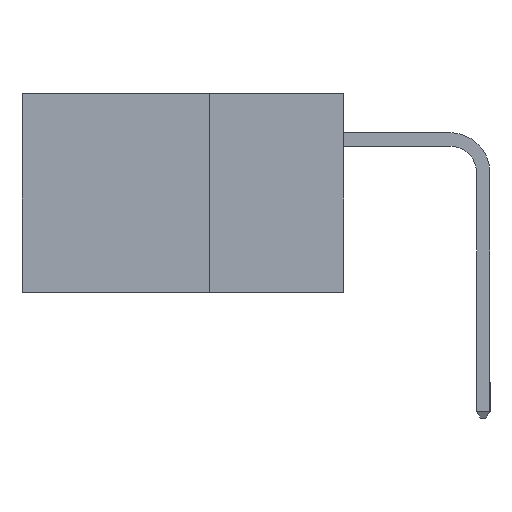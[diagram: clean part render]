
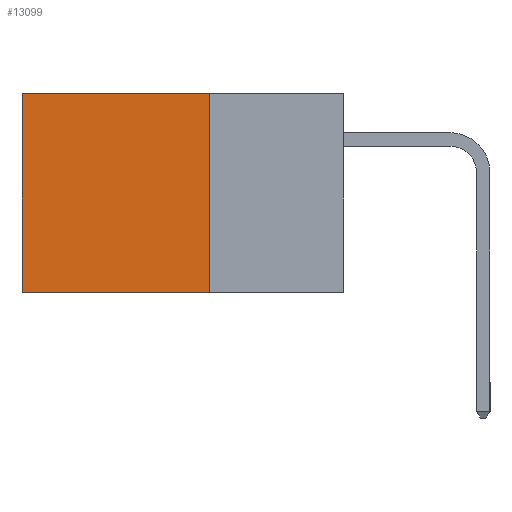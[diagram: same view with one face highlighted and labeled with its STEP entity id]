
A CAD part, left-side view. The second image highlights one B-rep face of the part: STEP entity #13099.
In plain terms, the highlighted planar face has unit normal (-1, 0, 0).
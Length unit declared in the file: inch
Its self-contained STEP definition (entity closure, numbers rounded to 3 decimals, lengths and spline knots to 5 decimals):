
#156 = DIRECTION ( 'NONE',  ( 0., 1., 0. ) ) ;
#207 = ORIENTED_EDGE ( 'NONE', *, *, #7930, .T. ) ;
#436 = ORIENTED_EDGE ( 'NONE', *, *, #2100, .F. ) ;
#729 = ORIENTED_EDGE ( 'NONE', *, *, #3779, .F. ) ;
#1089 = DIRECTION ( 'NONE',  ( 0., 0., -1. ) ) ;
#1371 = AXIS2_PLACEMENT_3D ( 'NONE', #12196, #5214, #13262 ) ;
#2100 = EDGE_CURVE ( 'NONE', #11274, #3250, #14864, .T. ) ;
#2381 = ORIENTED_EDGE ( 'NONE', *, *, #7625, .T. ) ;
#2775 = EDGE_LOOP ( 'NONE', ( #207, #436, #729, #2381 ) ) ;
#3250 = VERTEX_POINT ( 'NONE', #8927 ) ;
#3779 = EDGE_CURVE ( 'NONE', #6844, #11274, #8125, .T. ) ;
#3954 = PLANE ( 'NONE',  #1371 ) ;
#4610 = CARTESIAN_POINT ( 'NONE',  ( 0.298, 0.25, 0. ) ) ;
#5214 = DIRECTION ( 'NONE',  ( 1., 0., 0. ) ) ;
#5579 = CARTESIAN_POINT ( 'NONE',  ( 0.298, 0.6, 0. ) ) ;
#5842 = VECTOR ( 'NONE', #156, 39.37008 ) ;
#6231 = CARTESIAN_POINT ( 'NONE',  ( 0.298, 0.6, 0. ) ) ;
#6844 = VERTEX_POINT ( 'NONE', #4610 ) ;
#7481 = DIRECTION ( 'NONE',  ( 0., 1., 0. ) ) ;
#7625 = EDGE_CURVE ( 'NONE', #6844, #10869, #12028, .T. ) ;
#7738 = VECTOR ( 'NONE', #9317, 39.37008 ) ;
#7930 = EDGE_CURVE ( 'NONE', #10869, #3250, #11678, .T. ) ;
#8125 = LINE ( 'NONE', #10690, #7738 ) ;
#8489 = CARTESIAN_POINT ( 'NONE',  ( 0.298, 0.25, -0.37 ) ) ;
#8927 = CARTESIAN_POINT ( 'NONE',  ( 0.298, 0.6, -0.37 ) ) ;
#9141 = CARTESIAN_POINT ( 'NONE',  ( 0.298, 0.25, 0. ) ) ;
#9213 = VECTOR ( 'NONE', #7481, 39.37008 ) ;
#9317 = DIRECTION ( 'NONE',  ( 0., 0., -1. ) ) ;
#10690 = CARTESIAN_POINT ( 'NONE',  ( 0.298, 0.25, 0. ) ) ;
#10869 = VERTEX_POINT ( 'NONE', #5579 ) ;
#11274 = VERTEX_POINT ( 'NONE', #8489 ) ;
#11339 = VECTOR ( 'NONE', #1089, 39.37008 ) ;
#11678 = LINE ( 'NONE', #6231, #11339 ) ;
#12028 = LINE ( 'NONE', #9141, #5842 ) ;
#12196 = CARTESIAN_POINT ( 'NONE',  ( 0.298, 0.25, 0. ) ) ;
#13099 = ADVANCED_FACE ( 'NONE', ( #14546 ), #3954, .F. ) ;
#13262 = DIRECTION ( 'NONE',  ( 0., 0., -1. ) ) ;
#14331 = CARTESIAN_POINT ( 'NONE',  ( 0.298, 0.25, -0.37 ) ) ;
#14546 = FACE_OUTER_BOUND ( 'NONE', #2775, .T. ) ;
#14864 = LINE ( 'NONE', #14331, #9213 ) ;
